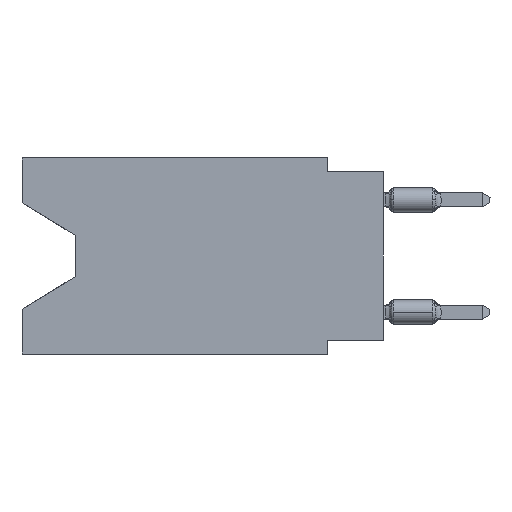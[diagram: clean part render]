
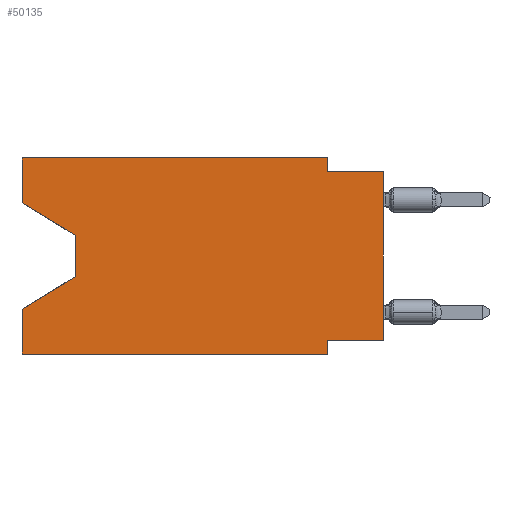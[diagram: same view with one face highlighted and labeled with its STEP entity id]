
A CAD part, left-side view. The second image highlights one B-rep face of the part: STEP entity #50135.
In plain terms, the highlighted planar face has unit normal (-1, 0, 0).
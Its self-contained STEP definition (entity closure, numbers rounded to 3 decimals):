
#3 = VECTOR ( 'NONE', #17374, 1000. ) ;
#938 = ORIENTED_EDGE ( 'NONE', *, *, #3841, .T. ) ;
#1914 = ORIENTED_EDGE ( 'NONE', *, *, #40846, .T. ) ;
#2094 = DIRECTION ( 'NONE',  ( 0., 0., -1. ) ) ;
#2332 = EDGE_CURVE ( 'NONE', #52171, #38814, #16822, .T. ) ;
#2389 = DIRECTION ( 'NONE',  ( 0., 1., 0. ) ) ;
#3149 = CARTESIAN_POINT ( 'NONE',  ( 0., 16.383, 0. ) ) ;
#3841 = EDGE_CURVE ( 'NONE', #36231, #38814, #39373, .T. ) ;
#3965 = CARTESIAN_POINT ( 'NONE',  ( 0., 16.383, 0. ) ) ;
#5168 = CARTESIAN_POINT ( 'NONE',  ( 0., 2.54, -8.89 ) ) ;
#5930 = CARTESIAN_POINT ( 'NONE',  ( 0., 0., -8.255 ) ) ;
#6518 = VECTOR ( 'NONE', #27867, 1000. ) ;
#7291 = VECTOR ( 'NONE', #37240, 1000. ) ;
#7425 = LINE ( 'NONE', #32166, #9820 ) ;
#9627 = DIRECTION ( 'NONE',  ( 0., 0.855, -0.519 ) ) ;
#9802 = VERTEX_POINT ( 'NONE', #14772 ) ;
#9820 = VECTOR ( 'NONE', #24004, 1000. ) ;
#11022 = DIRECTION ( 'NONE',  ( 1., 0., 0. ) ) ;
#11445 = CARTESIAN_POINT ( 'NONE',  ( 0., 0., -8.255 ) ) ;
#12880 = VERTEX_POINT ( 'NONE', #32689 ) ;
#13098 = CARTESIAN_POINT ( 'NONE',  ( 0., 2.54, -8.89 ) ) ;
#14772 = CARTESIAN_POINT ( 'NONE',  ( 0., 16.383, 0. ) ) ;
#14851 = EDGE_LOOP ( 'NONE', ( #21622, #1914, #44847, #19486, #31067, #51995, #45536, #938, #37132, #36117, #51214, #49590 ) ) ;
#14922 = CARTESIAN_POINT ( 'NONE',  ( 0., 13.97, -5.385 ) ) ;
#16048 = CARTESIAN_POINT ( 'NONE',  ( 0., 2.54, -0.635 ) ) ;
#16822 = LINE ( 'NONE', #20096, #7291 ) ;
#17374 = DIRECTION ( 'NONE',  ( 0., -1., 0. ) ) ;
#17532 = CARTESIAN_POINT ( 'NONE',  ( 0., 2.54, 0. ) ) ;
#18421 = EDGE_CURVE ( 'NONE', #36231, #45329, #30931, .T. ) ;
#18503 = VECTOR ( 'NONE', #20528, 1000. ) ;
#18706 = CARTESIAN_POINT ( 'NONE',  ( 0., 0., 0. ) ) ;
#19065 = CARTESIAN_POINT ( 'NONE',  ( 0., 0., -0.635 ) ) ;
#19408 = VECTOR ( 'NONE', #2389, 1000. ) ;
#19486 = ORIENTED_EDGE ( 'NONE', *, *, #47437, .F. ) ;
#20096 = CARTESIAN_POINT ( 'NONE',  ( 0., 0., -0.635 ) ) ;
#20366 = AXIS2_PLACEMENT_3D ( 'NONE', #3149, #11022, #48265 ) ;
#20528 = DIRECTION ( 'NONE',  ( 0., -1., 0. ) ) ;
#20659 = LINE ( 'NONE', #37257, #3 ) ;
#21622 = ORIENTED_EDGE ( 'NONE', *, *, #23398, .T. ) ;
#21746 = LINE ( 'NONE', #5168, #31764 ) ;
#22879 = VERTEX_POINT ( 'NONE', #14922 ) ;
#23398 = EDGE_CURVE ( 'NONE', #41248, #26531, #24102, .T. ) ;
#24004 = DIRECTION ( 'NONE',  ( 0., 0., -1. ) ) ;
#24102 = LINE ( 'NONE', #24905, #25845 ) ;
#24339 = FACE_OUTER_BOUND ( 'NONE', #14851, .T. ) ;
#24905 = CARTESIAN_POINT ( 'NONE',  ( 0., 16.383, -2.038 ) ) ;
#25027 = CARTESIAN_POINT ( 'NONE',  ( 0., 16.383, -8.89 ) ) ;
#25150 = LINE ( 'NONE', #3965, #18503 ) ;
#25845 = VECTOR ( 'NONE', #33342, 1000. ) ;
#26282 = CARTESIAN_POINT ( 'NONE',  ( 0., 13.97, -3.505 ) ) ;
#26379 = VECTOR ( 'NONE', #43983, 1000. ) ;
#26531 = VERTEX_POINT ( 'NONE', #33508 ) ;
#27867 = DIRECTION ( 'NONE',  ( 0., 0., 1. ) ) ;
#30694 = LINE ( 'NONE', #43738, #42040 ) ;
#30931 = LINE ( 'NONE', #5930, #19408 ) ;
#31067 = ORIENTED_EDGE ( 'NONE', *, *, #46012, .T. ) ;
#31764 = VECTOR ( 'NONE', #33976, 1000. ) ;
#32145 = VERTEX_POINT ( 'NONE', #17532 ) ;
#32166 = CARTESIAN_POINT ( 'NONE',  ( 0., 2.54, 0. ) ) ;
#32221 = LINE ( 'NONE', #35769, #6518 ) ;
#32689 = CARTESIAN_POINT ( 'NONE',  ( 0., 16.383, -6.852 ) ) ;
#32722 = VECTOR ( 'NONE', #2094, 1000. ) ;
#33342 = DIRECTION ( 'NONE',  ( 0., -0.855, -0.519 ) ) ;
#33508 = CARTESIAN_POINT ( 'NONE',  ( 0., 13.97, -3.505 ) ) ;
#33976 = DIRECTION ( 'NONE',  ( 0., 0., -1. ) ) ;
#34109 = VECTOR ( 'NONE', #9627, 1000. ) ;
#34126 = EDGE_CURVE ( 'NONE', #9802, #32145, #25150, .T. ) ;
#34359 = CARTESIAN_POINT ( 'NONE',  ( 0., 13.97, -5.385 ) ) ;
#34725 = LINE ( 'NONE', #26282, #32722 ) ;
#34784 = DIRECTION ( 'NONE',  ( 0., 0., 1. ) ) ;
#35769 = CARTESIAN_POINT ( 'NONE',  ( 0., 16.383, 0. ) ) ;
#36117 = ORIENTED_EDGE ( 'NONE', *, *, #48428, .F. ) ;
#36195 = VERTEX_POINT ( 'NONE', #25027 ) ;
#36231 = VERTEX_POINT ( 'NONE', #11445 ) ;
#36355 = EDGE_CURVE ( 'NONE', #45329, #48639, #21746, .T. ) ;
#37132 = ORIENTED_EDGE ( 'NONE', *, *, #2332, .F. ) ;
#37240 = DIRECTION ( 'NONE',  ( 0., -1., 0. ) ) ;
#37257 = CARTESIAN_POINT ( 'NONE',  ( 0., 16.383, -8.89 ) ) ;
#38161 = CARTESIAN_POINT ( 'NONE',  ( 0., 2.54, -8.255 ) ) ;
#38260 = EDGE_CURVE ( 'NONE', #22879, #12880, #38711, .T. ) ;
#38711 = LINE ( 'NONE', #34359, #34109 ) ;
#38814 = VERTEX_POINT ( 'NONE', #19065 ) ;
#39373 = LINE ( 'NONE', #18706, #26379 ) ;
#40846 = EDGE_CURVE ( 'NONE', #26531, #22879, #34725, .T. ) ;
#41248 = VERTEX_POINT ( 'NONE', #46882 ) ;
#42040 = VECTOR ( 'NONE', #34784, 1000. ) ;
#43738 = CARTESIAN_POINT ( 'NONE',  ( 0., 16.383, 0. ) ) ;
#43983 = DIRECTION ( 'NONE',  ( 0., 0., 1. ) ) ;
#44847 = ORIENTED_EDGE ( 'NONE', *, *, #38260, .T. ) ;
#45329 = VERTEX_POINT ( 'NONE', #38161 ) ;
#45536 = ORIENTED_EDGE ( 'NONE', *, *, #18421, .F. ) ;
#46012 = EDGE_CURVE ( 'NONE', #36195, #48639, #20659, .T. ) ;
#46882 = CARTESIAN_POINT ( 'NONE',  ( 0., 16.383, -2.038 ) ) ;
#47437 = EDGE_CURVE ( 'NONE', #36195, #12880, #30694, .T. ) ;
#48265 = DIRECTION ( 'NONE',  ( 0., 0., -1. ) ) ;
#48428 = EDGE_CURVE ( 'NONE', #32145, #52171, #7425, .T. ) ;
#48531 = PLANE ( 'NONE',  #20366 ) ;
#48639 = VERTEX_POINT ( 'NONE', #13098 ) ;
#49590 = ORIENTED_EDGE ( 'NONE', *, *, #50222, .F. ) ;
#50135 = ADVANCED_FACE ( 'NONE', ( #24339 ), #48531, .F. ) ;
#50222 = EDGE_CURVE ( 'NONE', #41248, #9802, #32221, .T. ) ;
#51214 = ORIENTED_EDGE ( 'NONE', *, *, #34126, .F. ) ;
#51995 = ORIENTED_EDGE ( 'NONE', *, *, #36355, .F. ) ;
#52171 = VERTEX_POINT ( 'NONE', #16048 ) ;
